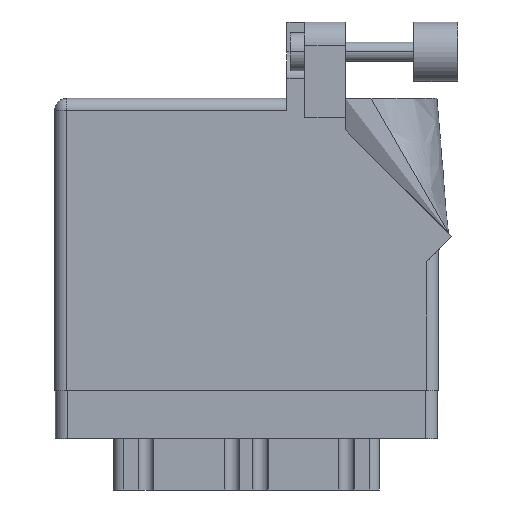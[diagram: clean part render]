
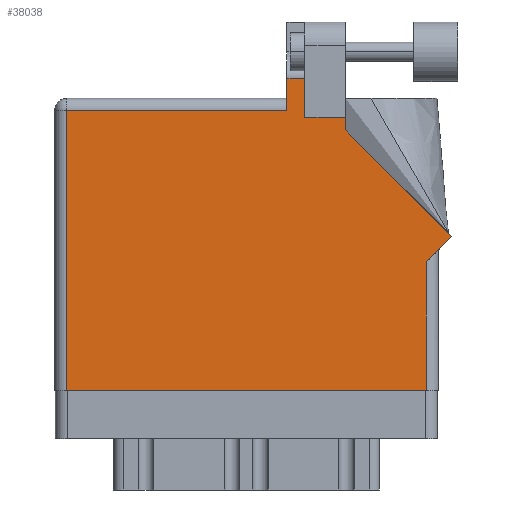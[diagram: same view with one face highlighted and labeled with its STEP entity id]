
A CAD part, front view. The second image highlights one B-rep face of the part: STEP entity #38038.
In plain terms, the highlighted face is planar.
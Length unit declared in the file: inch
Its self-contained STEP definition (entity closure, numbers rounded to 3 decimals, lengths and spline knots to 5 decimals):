
#277 = DIRECTION ( 'NONE',  ( 0., -1., 0. ) ) ;
#414 = VERTEX_POINT ( 'NONE', #26639 ) ;
#933 = DIRECTION ( 'NONE',  ( -0.707, 0.707, 0. ) ) ;
#1032 = ORIENTED_EDGE ( 'NONE', *, *, #38203, .T. ) ;
#1617 = CARTESIAN_POINT ( 'NONE',  ( 1.524, 1.36442, 0. ) ) ;
#3265 = CARTESIAN_POINT ( 'NONE',  ( 2.01, 0.737, 0. ) ) ;
#3440 = CARTESIAN_POINT ( 'NONE',  ( 1.524, 1.43, 0. ) ) ;
#3495 = VERTEX_POINT ( 'NONE', #3440 ) ;
#3635 = VECTOR ( 'NONE', #31140, 39.37008 ) ;
#3944 = ORIENTED_EDGE ( 'NONE', *, *, #27066, .T. ) ;
#5405 = CARTESIAN_POINT ( 'NONE',  ( 2.08071, 0.80771, 0. ) ) ;
#5581 = VECTOR ( 'NONE', #20597, 39.37008 ) ;
#5979 = EDGE_CURVE ( 'NONE', #25206, #16840, #34265, .T. ) ;
#6147 = AXIS2_PLACEMENT_3D ( 'NONE', #37706, #7643, #22445 ) ;
#6487 = LINE ( 'NONE', #21676, #21640 ) ;
#6518 = EDGE_CURVE ( 'NONE', #414, #18393, #10298, .T. ) ;
#6644 = CARTESIAN_POINT ( 'NONE',  ( 2.08071, 0.80771, 0. ) ) ;
#6958 = CARTESIAN_POINT ( 'NONE',  ( 1.524, 1.36442, 0. ) ) ;
#7181 = CARTESIAN_POINT ( 'NONE',  ( 1.311, 1.43, 0. ) ) ;
#7285 = CARTESIAN_POINT ( 'NONE',  ( 0.062, 0., 0. ) ) ;
#7463 = EDGE_CURVE ( 'NONE', #8918, #18799, #27317, .T. ) ;
#7643 = DIRECTION ( 'NONE',  ( 0., 0., -1. ) ) ;
#8918 = VERTEX_POINT ( 'NONE', #15909 ) ;
#9391 = DIRECTION ( 'NONE',  ( 0., 1., 0. ) ) ;
#9431 = LINE ( 'NONE', #6644, #34702 ) ;
#9469 = ORIENTED_EDGE ( 'NONE', *, *, #29759, .T. ) ;
#9473 = VERTEX_POINT ( 'NONE', #1617 ) ;
#9834 = ORIENTED_EDGE ( 'NONE', *, *, #10174, .T. ) ;
#9882 = ORIENTED_EDGE ( 'NONE', *, *, #7463, .T. ) ;
#10174 = EDGE_CURVE ( 'NONE', #18393, #8918, #19837, .T. ) ;
#10298 = LINE ( 'NONE', #19378, #12508 ) ;
#10413 = FACE_OUTER_BOUND ( 'NONE', #27399, .T. ) ;
#12508 = VECTOR ( 'NONE', #29614, 39.37008 ) ;
#12796 = EDGE_CURVE ( 'NONE', #18799, #35718, #6487, .T. ) ;
#12864 = VERTEX_POINT ( 'NONE', #24853 ) ;
#13319 = CARTESIAN_POINT ( 'NONE',  ( 1.311, 1.6315, 0. ) ) ;
#13560 = EDGE_CURVE ( 'NONE', #3495, #25206, #22666, .T. ) ;
#13979 = VERTEX_POINT ( 'NONE', #5405 ) ;
#14106 = CARTESIAN_POINT ( 'NONE',  ( 1.64177, 1.6315, 0. ) ) ;
#14250 = CARTESIAN_POINT ( 'NONE',  ( 1.217, 1.468, 0. ) ) ;
#14857 = ORIENTED_EDGE ( 'NONE', *, *, #12796, .T. ) ;
#15674 = DIRECTION ( 'NONE',  ( 0., 1., 0. ) ) ;
#15909 = CARTESIAN_POINT ( 'NONE',  ( 0.062, 1.468, 0. ) ) ;
#16108 = CARTESIAN_POINT ( 'NONE',  ( 0., 1.468, 0. ) ) ;
#16286 = EDGE_CURVE ( 'NONE', #13979, #9473, #9431, .T. ) ;
#16441 = CARTESIAN_POINT ( 'NONE',  ( 1.948, 0., 0. ) ) ;
#16840 = VERTEX_POINT ( 'NONE', #13319 ) ;
#18174 = DIRECTION ( 'NONE',  ( 1., 0., 0. ) ) ;
#18393 = VERTEX_POINT ( 'NONE', #14250 ) ;
#18535 = ORIENTED_EDGE ( 'NONE', *, *, #16286, .T. ) ;
#18799 = VERTEX_POINT ( 'NONE', #7285 ) ;
#18971 = ORIENTED_EDGE ( 'NONE', *, *, #13560, .T. ) ;
#19378 = CARTESIAN_POINT ( 'NONE',  ( 1.217, 1.53, 0. ) ) ;
#19837 = LINE ( 'NONE', #16108, #38312 ) ;
#20597 = DIRECTION ( 'NONE',  ( -1., 0., 0. ) ) ;
#20688 = ORIENTED_EDGE ( 'NONE', *, *, #23764, .T. ) ;
#21640 = VECTOR ( 'NONE', #18174, 39.37008 ) ;
#21676 = CARTESIAN_POINT ( 'NONE',  ( 0., 0., 0. ) ) ;
#21796 = LINE ( 'NONE', #3265, #32544 ) ;
#21880 = DIRECTION ( 'NONE',  ( -1., 0., 0. ) ) ;
#22008 = DIRECTION ( 'NONE',  ( -1., 0., 0. ) ) ;
#22017 = LINE ( 'NONE', #34098, #3635 ) ;
#22445 = DIRECTION ( 'NONE',  ( -1., 0., 0. ) ) ;
#22666 = LINE ( 'NONE', #34753, #30342 ) ;
#23458 = ORIENTED_EDGE ( 'NONE', *, *, #5979, .T. ) ;
#23764 = EDGE_CURVE ( 'NONE', #12864, #13979, #21796, .T. ) ;
#24853 = CARTESIAN_POINT ( 'NONE',  ( 1.948, 0.675, 0. ) ) ;
#25206 = VERTEX_POINT ( 'NONE', #28540 ) ;
#25621 = PLANE ( 'NONE',  #6147 ) ;
#26639 = CARTESIAN_POINT ( 'NONE',  ( 1.217, 1.6315, 0. ) ) ;
#27066 = EDGE_CURVE ( 'NONE', #16840, #414, #32287, .T. ) ;
#27317 = LINE ( 'NONE', #32885, #28377 ) ;
#27359 = DIRECTION ( 'NONE',  ( 0.707, 0.707, 0. ) ) ;
#27399 = EDGE_LOOP ( 'NONE', ( #23458, #3944, #28772, #9834, #9882, #14857, #1032, #20688, #18535, #9469, #18971 ) ) ;
#28377 = VECTOR ( 'NONE', #277, 39.37008 ) ;
#28540 = CARTESIAN_POINT ( 'NONE',  ( 1.311, 1.43, 0. ) ) ;
#28772 = ORIENTED_EDGE ( 'NONE', *, *, #6518, .T. ) ;
#29614 = DIRECTION ( 'NONE',  ( 0., -1., 0. ) ) ;
#29759 = EDGE_CURVE ( 'NONE', #9473, #3495, #37018, .T. ) ;
#30342 = VECTOR ( 'NONE', #21880, 39.37008 ) ;
#31140 = DIRECTION ( 'NONE',  ( 0., 1., 0. ) ) ;
#32287 = LINE ( 'NONE', #14106, #5581 ) ;
#32544 = VECTOR ( 'NONE', #27359, 39.37008 ) ;
#32885 = CARTESIAN_POINT ( 'NONE',  ( 0.062, 0., 0. ) ) ;
#33309 = VECTOR ( 'NONE', #9391, 39.37008 ) ;
#34098 = CARTESIAN_POINT ( 'NONE',  ( 1.948, 0.737, 0. ) ) ;
#34265 = LINE ( 'NONE', #7181, #33309 ) ;
#34702 = VECTOR ( 'NONE', #933, 39.37008 ) ;
#34753 = CARTESIAN_POINT ( 'NONE',  ( 1.524, 1.43, 0. ) ) ;
#35718 = VERTEX_POINT ( 'NONE', #16441 ) ;
#36683 = VECTOR ( 'NONE', #15674, 39.37008 ) ;
#37018 = LINE ( 'NONE', #6958, #36683 ) ;
#37706 = CARTESIAN_POINT ( 'NONE',  ( 0., 1.53, 0. ) ) ;
#38038 = ADVANCED_FACE ( 'NONE', ( #10413 ), #25621, .F. ) ;
#38203 = EDGE_CURVE ( 'NONE', #35718, #12864, #22017, .T. ) ;
#38312 = VECTOR ( 'NONE', #22008, 39.37008 ) ;
